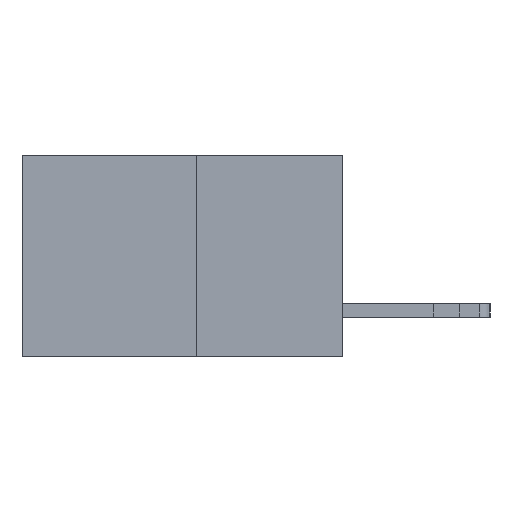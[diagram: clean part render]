
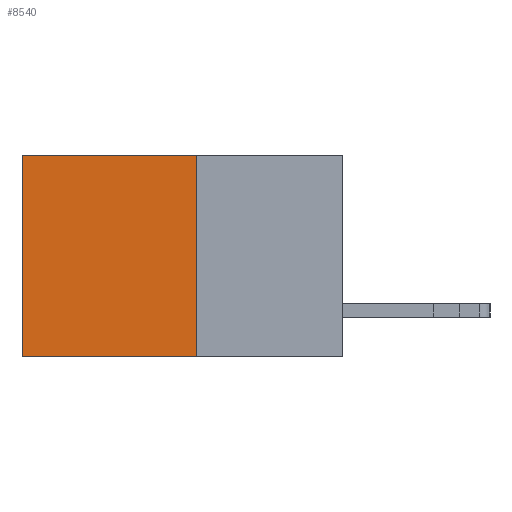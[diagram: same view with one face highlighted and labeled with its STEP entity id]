
A CAD part, left-side view. The second image highlights one B-rep face of the part: STEP entity #8540.
In plain terms, the highlighted planar face has unit normal (-1, 0, 0).
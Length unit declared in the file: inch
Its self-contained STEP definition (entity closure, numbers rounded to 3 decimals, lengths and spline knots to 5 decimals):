
#833 = CARTESIAN_POINT ( 'NONE',  ( 0.277, 0.27, 0. ) ) ;
#1063 = PLANE ( 'NONE',  #19884 ) ;
#3802 = VECTOR ( 'NONE', #20136, 39.37008 ) ;
#4219 = EDGE_CURVE ( 'NONE', #21367, #22542, #7958, .T. ) ;
#5332 = CARTESIAN_POINT ( 'NONE',  ( 0.277, 0.59, -0.37 ) ) ;
#5573 = EDGE_CURVE ( 'NONE', #10808, #12254, #12207, .T. ) ;
#6417 = VECTOR ( 'NONE', #6966, 39.37008 ) ;
#6966 = DIRECTION ( 'NONE',  ( 0., 0., -1. ) ) ;
#7592 = ORIENTED_EDGE ( 'NONE', *, *, #11270, .F. ) ;
#7617 = ORIENTED_EDGE ( 'NONE', *, *, #16519, .T. ) ;
#7958 = LINE ( 'NONE', #833, #3802 ) ;
#8188 = VECTOR ( 'NONE', #19198, 39.37008 ) ;
#8199 = VECTOR ( 'NONE', #18338, 39.37008 ) ;
#8540 = ADVANCED_FACE ( 'NONE', ( #21949 ), #1063, .F. ) ;
#8722 = LINE ( 'NONE', #5332, #8188 ) ;
#9250 = ORIENTED_EDGE ( 'NONE', *, *, #5573, .F. ) ;
#9645 = CARTESIAN_POINT ( 'NONE',  ( 0.277, 0.27, -0.37 ) ) ;
#10004 = DIRECTION ( 'NONE',  ( 0., 0., -1. ) ) ;
#10808 = VERTEX_POINT ( 'NONE', #16077 ) ;
#11270 = EDGE_CURVE ( 'NONE', #21367, #10808, #15540, .T. ) ;
#12207 = LINE ( 'NONE', #9645, #8199 ) ;
#12254 = VERTEX_POINT ( 'NONE', #13368 ) ;
#12711 = EDGE_LOOP ( 'NONE', ( #7617, #9250, #7592, #15521 ) ) ;
#13368 = CARTESIAN_POINT ( 'NONE',  ( 0.277, 0.59, -0.37 ) ) ;
#14245 = CARTESIAN_POINT ( 'NONE',  ( 0.277, 0.59, 0. ) ) ;
#15521 = ORIENTED_EDGE ( 'NONE', *, *, #4219, .T. ) ;
#15540 = LINE ( 'NONE', #17261, #6417 ) ;
#16077 = CARTESIAN_POINT ( 'NONE',  ( 0.277, 0.27, -0.37 ) ) ;
#16519 = EDGE_CURVE ( 'NONE', #22542, #12254, #8722, .T. ) ;
#16834 = CARTESIAN_POINT ( 'NONE',  ( 0.277, 0.27, -0.37 ) ) ;
#17261 = CARTESIAN_POINT ( 'NONE',  ( 0.277, 0.27, -0.37 ) ) ;
#18338 = DIRECTION ( 'NONE',  ( 0., 1., 0. ) ) ;
#19198 = DIRECTION ( 'NONE',  ( 0., 0., -1. ) ) ;
#19598 = CARTESIAN_POINT ( 'NONE',  ( 0.277, 0.27, 0. ) ) ;
#19884 = AXIS2_PLACEMENT_3D ( 'NONE', #16834, #20444, #10004 ) ;
#20136 = DIRECTION ( 'NONE',  ( 0., 1., 0. ) ) ;
#20444 = DIRECTION ( 'NONE',  ( 1., 0., 0. ) ) ;
#21367 = VERTEX_POINT ( 'NONE', #19598 ) ;
#21949 = FACE_OUTER_BOUND ( 'NONE', #12711, .T. ) ;
#22542 = VERTEX_POINT ( 'NONE', #14245 ) ;
